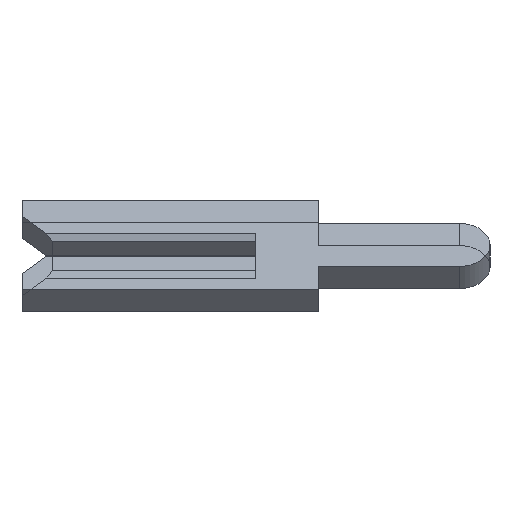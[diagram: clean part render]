
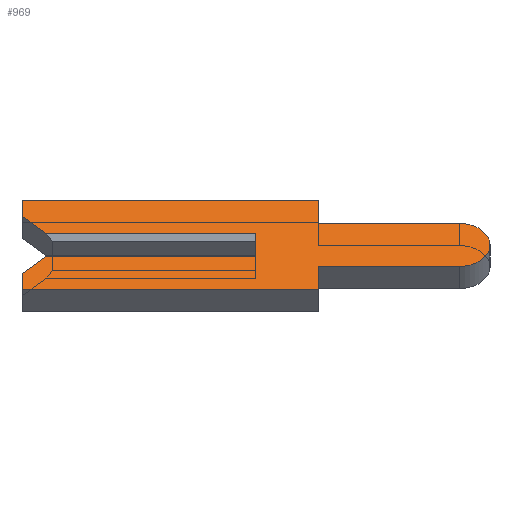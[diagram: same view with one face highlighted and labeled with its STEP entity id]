
A CAD part, left-side view. The second image highlights one B-rep face of the part: STEP entity #969.
In plain terms, the highlighted face is planar.
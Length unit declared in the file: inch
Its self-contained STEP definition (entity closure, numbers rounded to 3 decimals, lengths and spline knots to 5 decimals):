
#13 = DIRECTION ( 'NONE',  ( 0., 1., 0. ) ) ;
#46 = CARTESIAN_POINT ( 'NONE',  ( -0.01, 0.15, -0.026 ) ) ;
#182 = CARTESIAN_POINT ( 'NONE',  ( -0.01, -0.04, -0.04 ) ) ;
#210 = VERTEX_POINT ( 'NONE', #2328 ) ;
#289 = DIRECTION ( 'NONE',  ( 0., -1., 0. ) ) ;
#315 = CARTESIAN_POINT ( 'NONE',  ( -0.01, 0.15, 0.026 ) ) ;
#318 = EDGE_CURVE ( 'NONE', #210, #2918, #922, .T. ) ;
#319 = VERTEX_POINT ( 'NONE', #1006 ) ;
#351 = CARTESIAN_POINT ( 'NONE',  ( -0.01, 0.15, -0.026 ) ) ;
#386 = ORIENTED_EDGE ( 'NONE', *, *, #2093, .F. ) ;
#401 = VECTOR ( 'NONE', #3101, 39.37008 ) ;
#426 = DIRECTION ( 'NONE',  ( 0., 0., -1. ) ) ;
#456 = EDGE_CURVE ( 'NONE', #2735, #3064, #1844, .T. ) ;
#480 = LINE ( 'NONE', #1540, #3232 ) ;
#484 = CARTESIAN_POINT ( 'NONE',  ( -0.01, -0.04, 0.04 ) ) ;
#514 = LINE ( 'NONE', #1661, #3402 ) ;
#528 = CARTESIAN_POINT ( 'NONE',  ( -0.01, 0.1305, -0.0065 ) ) ;
#544 = VECTOR ( 'NONE', #1351, 39.37008 ) ;
#596 = DIRECTION ( 'NONE',  ( 0., 0., 1. ) ) ;
#603 = VERTEX_POINT ( 'NONE', #2649 ) ;
#634 = CIRCLE ( 'NONE', #3436, 0.0195 ) ;
#639 = LINE ( 'NONE', #3337, #811 ) ;
#649 = ORIENTED_EDGE ( 'NONE', *, *, #2327, .F. ) ;
#653 = VERTEX_POINT ( 'NONE', #182 ) ;
#697 = EDGE_CURVE ( 'NONE', #2008, #1275, #480, .T. ) ;
#733 = ORIENTED_EDGE ( 'NONE', *, *, #2238, .F. ) ;
#735 = CARTESIAN_POINT ( 'NONE',  ( -0.01, -0.1305, 0. ) ) ;
#811 = VECTOR ( 'NONE', #13, 39.37008 ) ;
#887 = ORIENTED_EDGE ( 'NONE', *, *, #2916, .F. ) ;
#922 = LINE ( 'NONE', #3199, #2704 ) ;
#933 = CARTESIAN_POINT ( 'NONE',  ( -0.01, 0.134, -0.01 ) ) ;
#969 = ADVANCED_FACE ( 'NONE', ( #3324 ), #3513, .F. ) ;
#1006 = CARTESIAN_POINT ( 'NONE',  ( -0.01, -0.1305, 0.0195 ) ) ;
#1016 = CARTESIAN_POINT ( 'NONE',  ( -0.01, -0.1305, -0.01 ) ) ;
#1076 = LINE ( 'NONE', #3052, #544 ) ;
#1259 = EDGE_CURVE ( 'NONE', #3146, #3090, #2887, .T. ) ;
#1268 = CARTESIAN_POINT ( 'NONE',  ( -0.01, 0.15, 0.01 ) ) ;
#1275 = VERTEX_POINT ( 'NONE', #1593 ) ;
#1291 = VECTOR ( 'NONE', #596, 39.37008 ) ;
#1351 = DIRECTION ( 'NONE',  ( 0., 0., -1. ) ) ;
#1358 = CARTESIAN_POINT ( 'NONE',  ( -0.01, 0.15, 0.04 ) ) ;
#1449 = CARTESIAN_POINT ( 'NONE',  ( -0.01, 0., -0.01 ) ) ;
#1464 = LINE ( 'NONE', #484, #2858 ) ;
#1475 = CARTESIAN_POINT ( 'NONE',  ( -0.01, 0., 0.0065 ) ) ;
#1540 = CARTESIAN_POINT ( 'NONE',  ( -0.01, 0.15, 0.04 ) ) ;
#1578 = DIRECTION ( 'NONE',  ( 0., -1., 0. ) ) ;
#1593 = CARTESIAN_POINT ( 'NONE',  ( -0.01, -0.04, 0.04 ) ) ;
#1605 = ORIENTED_EDGE ( 'NONE', *, *, #1815, .F. ) ;
#1661 = CARTESIAN_POINT ( 'NONE',  ( -0.01, -0.04, 0.0195 ) ) ;
#1706 = CARTESIAN_POINT ( 'NONE',  ( -0.01, 0.15, -0.04 ) ) ;
#1711 = LINE ( 'NONE', #315, #401 ) ;
#1728 = CARTESIAN_POINT ( 'NONE',  ( -0.01, -0.04, -0.0195 ) ) ;
#1750 = VECTOR ( 'NONE', #3286, 39.37008 ) ;
#1815 = EDGE_CURVE ( 'NONE', #1275, #3494, #1464, .T. ) ;
#1842 = CARTESIAN_POINT ( 'NONE',  ( -0.01, -0.1305, 0. ) ) ;
#1844 = LINE ( 'NONE', #1268, #1931 ) ;
#1888 = EDGE_CURVE ( 'NONE', #2918, #653, #1076, .T. ) ;
#1931 = VECTOR ( 'NONE', #2140, 39.37008 ) ;
#2002 = ORIENTED_EDGE ( 'NONE', *, *, #697, .F. ) ;
#2008 = VERTEX_POINT ( 'NONE', #1358 ) ;
#2033 = LINE ( 'NONE', #3367, #2122 ) ;
#2093 = EDGE_CURVE ( 'NONE', #2923, #3146, #2658, .T. ) ;
#2122 = VECTOR ( 'NONE', #2790, 39.37008 ) ;
#2133 = ORIENTED_EDGE ( 'NONE', *, *, #2217, .F. ) ;
#2140 = DIRECTION ( 'NONE',  ( 0., -1., 0. ) ) ;
#2217 = EDGE_CURVE ( 'NONE', #2735, #603, #2033, .T. ) ;
#2238 = EDGE_CURVE ( 'NONE', #2564, #2923, #2768, .T. ) ;
#2327 = EDGE_CURVE ( 'NONE', #3494, #319, #514, .T. ) ;
#2328 = CARTESIAN_POINT ( 'NONE',  ( -0.01, -0.1305, -0.0195 ) ) ;
#2393 = DIRECTION ( 'NONE',  ( 1., 0., 0. ) ) ;
#2439 = DIRECTION ( 'NONE',  ( 0., 0., -1. ) ) ;
#2443 = EDGE_CURVE ( 'NONE', #653, #2564, #639, .T. ) ;
#2564 = VERTEX_POINT ( 'NONE', #1706 ) ;
#2570 = VECTOR ( 'NONE', #2973, 39.37008 ) ;
#2587 = DIRECTION ( 'NONE',  ( 0., 1., 0. ) ) ;
#2641 = LINE ( 'NONE', #1475, #3194 ) ;
#2643 = ORIENTED_EDGE ( 'NONE', *, *, #2794, .F. ) ;
#2649 = CARTESIAN_POINT ( 'NONE',  ( -0.01, 0.15, 0.026 ) ) ;
#2658 = LINE ( 'NONE', #528, #1750 ) ;
#2704 = VECTOR ( 'NONE', #2587, 39.37008 ) ;
#2735 = VERTEX_POINT ( 'NONE', #3094 ) ;
#2752 = ORIENTED_EDGE ( 'NONE', *, *, #456, .T. ) ;
#2768 = LINE ( 'NONE', #46, #1291 ) ;
#2783 = ORIENTED_EDGE ( 'NONE', *, *, #318, .F. ) ;
#2790 = DIRECTION ( 'NONE',  ( 0., 0.707, 0.707 ) ) ;
#2794 = EDGE_CURVE ( 'NONE', #603, #2008, #1711, .T. ) ;
#2831 = ORIENTED_EDGE ( 'NONE', *, *, #2443, .F. ) ;
#2849 = EDGE_LOOP ( 'NONE', ( #2752, #887, #3238, #386, #733, #2831, #3268, #2783, #3190, #649, #1605, #2002, #2643, #2133 ) ) ;
#2858 = VECTOR ( 'NONE', #2439, 39.37008 ) ;
#2861 = DIRECTION ( 'NONE',  ( 0., 0., 1. ) ) ;
#2887 = LINE ( 'NONE', #1016, #2570 ) ;
#2916 = EDGE_CURVE ( 'NONE', #3090, #3064, #2641, .T. ) ;
#2918 = VERTEX_POINT ( 'NONE', #1728 ) ;
#2923 = VERTEX_POINT ( 'NONE', #351 ) ;
#2941 = DIRECTION ( 'NONE',  ( 0., 0., -1. ) ) ;
#2973 = DIRECTION ( 'NONE',  ( 0., -1., 0. ) ) ;
#3052 = CARTESIAN_POINT ( 'NONE',  ( -0.01, -0.04, -0.04 ) ) ;
#3064 = VERTEX_POINT ( 'NONE', #3143 ) ;
#3090 = VERTEX_POINT ( 'NONE', #1449 ) ;
#3094 = CARTESIAN_POINT ( 'NONE',  ( -0.01, 0.134, 0.01 ) ) ;
#3101 = DIRECTION ( 'NONE',  ( 0., 0., 1. ) ) ;
#3143 = CARTESIAN_POINT ( 'NONE',  ( -0.01, 0., 0.01 ) ) ;
#3146 = VERTEX_POINT ( 'NONE', #933 ) ;
#3190 = ORIENTED_EDGE ( 'NONE', *, *, #3385, .F. ) ;
#3194 = VECTOR ( 'NONE', #2861, 39.37008 ) ;
#3199 = CARTESIAN_POINT ( 'NONE',  ( -0.01, -0.04, -0.0195 ) ) ;
#3217 = CARTESIAN_POINT ( 'NONE',  ( -0.01, -0.04, 0.0195 ) ) ;
#3232 = VECTOR ( 'NONE', #1578, 39.37008 ) ;
#3237 = DIRECTION ( 'NONE',  ( 1., 0., 0. ) ) ;
#3238 = ORIENTED_EDGE ( 'NONE', *, *, #1259, .F. ) ;
#3266 = AXIS2_PLACEMENT_3D ( 'NONE', #1842, #3237, #426 ) ;
#3268 = ORIENTED_EDGE ( 'NONE', *, *, #1888, .F. ) ;
#3286 = DIRECTION ( 'NONE',  ( 0., -0.707, 0.707 ) ) ;
#3324 = FACE_OUTER_BOUND ( 'NONE', #2849, .T. ) ;
#3337 = CARTESIAN_POINT ( 'NONE',  ( -0.01, 0.15, -0.04 ) ) ;
#3367 = CARTESIAN_POINT ( 'NONE',  ( -0.01, 0.1305, 0.0065 ) ) ;
#3385 = EDGE_CURVE ( 'NONE', #319, #210, #634, .T. ) ;
#3402 = VECTOR ( 'NONE', #289, 39.37008 ) ;
#3436 = AXIS2_PLACEMENT_3D ( 'NONE', #735, #2393, #2941 ) ;
#3494 = VERTEX_POINT ( 'NONE', #3217 ) ;
#3513 = PLANE ( 'NONE',  #3266 ) ;
